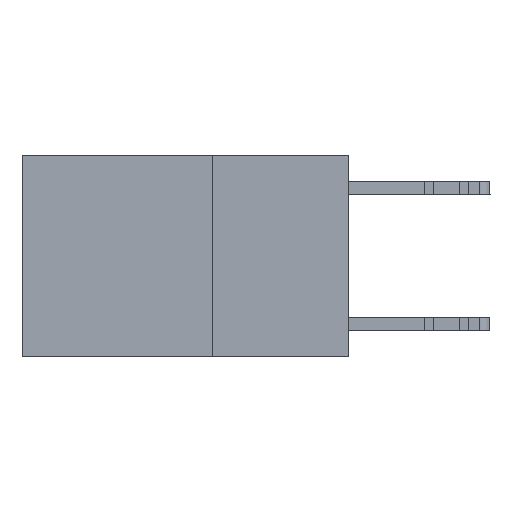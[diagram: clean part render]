
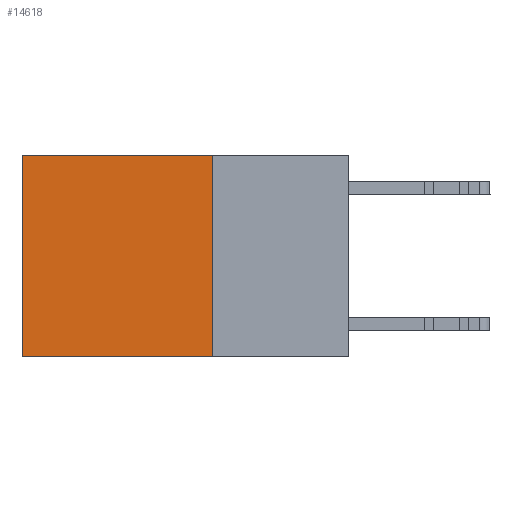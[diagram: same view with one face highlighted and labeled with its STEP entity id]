
A CAD part, left-side view. The second image highlights one B-rep face of the part: STEP entity #14618.
In plain terms, the highlighted planar face has unit normal (-1, 0, 0).
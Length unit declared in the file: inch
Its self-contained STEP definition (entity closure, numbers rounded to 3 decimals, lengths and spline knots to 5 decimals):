
#83 = DIRECTION ( 'NONE',  ( 0., 1., 0. ) ) ;
#137 = ORIENTED_EDGE ( 'NONE', *, *, #22064, .T. ) ;
#933 = EDGE_CURVE ( 'NONE', #21560, #5468, #17775, .T. ) ;
#2019 = CARTESIAN_POINT ( 'NONE',  ( 0.2625, 0.25, 0. ) ) ;
#2324 = CARTESIAN_POINT ( 'NONE',  ( 0.2625, 0.25, -0.37 ) ) ;
#3271 = VECTOR ( 'NONE', #5486, 39.37008 ) ;
#4372 = AXIS2_PLACEMENT_3D ( 'NONE', #18037, #17938, #17914 ) ;
#5114 = FACE_OUTER_BOUND ( 'NONE', #23751, .T. ) ;
#5468 = VERTEX_POINT ( 'NONE', #12919 ) ;
#5486 = DIRECTION ( 'NONE',  ( 0., 0., -1. ) ) ;
#5744 = CARTESIAN_POINT ( 'NONE',  ( 0.2625, 0.25, 0. ) ) ;
#5896 = ORIENTED_EDGE ( 'NONE', *, *, #29432, .F. ) ;
#5902 = EDGE_CURVE ( 'NONE', #24641, #5468, #25230, .T. ) ;
#5985 = VECTOR ( 'NONE', #8095, 39.37008 ) ;
#6233 = LINE ( 'NONE', #5744, #5985 ) ;
#8095 = DIRECTION ( 'NONE',  ( 0., 1., 0. ) ) ;
#9476 = LINE ( 'NONE', #21493, #3271 ) ;
#12919 = CARTESIAN_POINT ( 'NONE',  ( 0.2625, 0.6, -0.37 ) ) ;
#14436 = CARTESIAN_POINT ( 'NONE',  ( 0.2625, 0.25, -0.37 ) ) ;
#14618 = ADVANCED_FACE ( 'NONE', ( #5114 ), #18070, .F. ) ;
#17738 = VECTOR ( 'NONE', #83, 39.37008 ) ;
#17775 = LINE ( 'NONE', #2324, #17738 ) ;
#17914 = DIRECTION ( 'NONE',  ( 0., 0., -1. ) ) ;
#17938 = DIRECTION ( 'NONE',  ( 1., 0., 0. ) ) ;
#17974 = ORIENTED_EDGE ( 'NONE', *, *, #933, .F. ) ;
#18037 = CARTESIAN_POINT ( 'NONE',  ( 0.2625, 0.25, 0. ) ) ;
#18070 = PLANE ( 'NONE',  #4372 ) ;
#21493 = CARTESIAN_POINT ( 'NONE',  ( 0.2625, 0.25, 0. ) ) ;
#21560 = VERTEX_POINT ( 'NONE', #14436 ) ;
#21721 = CARTESIAN_POINT ( 'NONE',  ( 0.2625, 0.6, 0. ) ) ;
#22064 = EDGE_CURVE ( 'NONE', #23024, #24641, #6233, .T. ) ;
#23024 = VERTEX_POINT ( 'NONE', #2019 ) ;
#23751 = EDGE_LOOP ( 'NONE', ( #25308, #17974, #5896, #137 ) ) ;
#24641 = VERTEX_POINT ( 'NONE', #21721 ) ;
#25057 = VECTOR ( 'NONE', #27388, 39.37008 ) ;
#25230 = LINE ( 'NONE', #27848, #25057 ) ;
#25308 = ORIENTED_EDGE ( 'NONE', *, *, #5902, .T. ) ;
#27388 = DIRECTION ( 'NONE',  ( 0., 0., -1. ) ) ;
#27848 = CARTESIAN_POINT ( 'NONE',  ( 0.2625, 0.6, 0. ) ) ;
#29432 = EDGE_CURVE ( 'NONE', #23024, #21560, #9476, .T. ) ;
